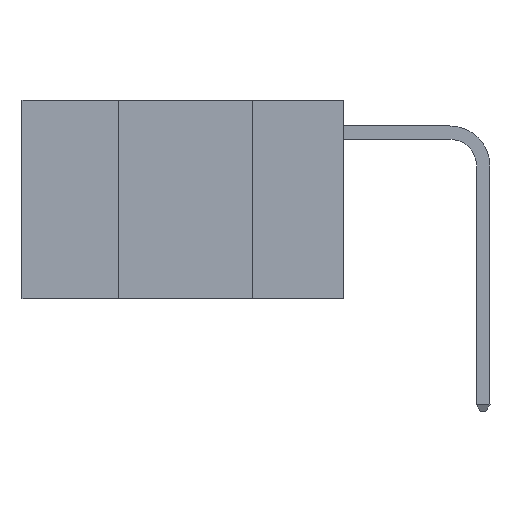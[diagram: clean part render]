
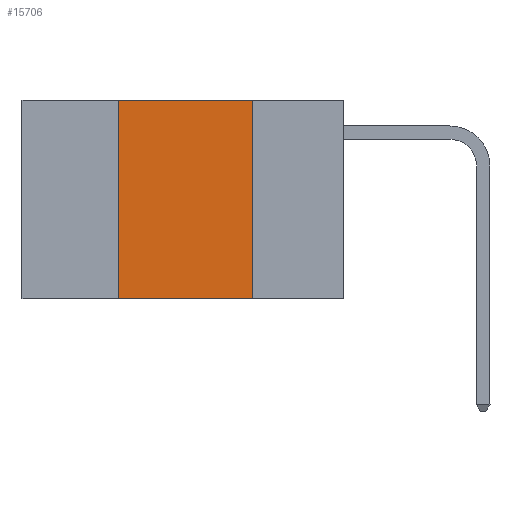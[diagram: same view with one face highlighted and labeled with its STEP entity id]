
A CAD part, left-side view. The second image highlights one B-rep face of the part: STEP entity #15706.
In plain terms, the highlighted planar face has unit normal (-1, 0, 0).
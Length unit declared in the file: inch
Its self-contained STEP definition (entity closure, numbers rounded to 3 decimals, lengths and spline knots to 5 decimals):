
#276 = DIRECTION ( 'NONE',  ( 0., 0., -1. ) ) ;
#886 = CARTESIAN_POINT ( 'NONE',  ( 0., 0.42, 0. ) ) ;
#909 = EDGE_LOOP ( 'NONE', ( #3582, #3209, #13281, #2622 ) ) ;
#1167 = DIRECTION ( 'NONE',  ( 0., -1., 0. ) ) ;
#1270 = LINE ( 'NONE', #5853, #17701 ) ;
#1848 = EDGE_CURVE ( 'NONE', #11623, #16429, #11668, .T. ) ;
#2243 = DIRECTION ( 'NONE',  ( 1., 0., 0. ) ) ;
#2622 = ORIENTED_EDGE ( 'NONE', *, *, #12399, .T. ) ;
#3209 = ORIENTED_EDGE ( 'NONE', *, *, #17516, .F. ) ;
#3312 = VECTOR ( 'NONE', #17788, 39.37008 ) ;
#3582 = ORIENTED_EDGE ( 'NONE', *, *, #1848, .F. ) ;
#3611 = VERTEX_POINT ( 'NONE', #13261 ) ;
#3947 = DIRECTION ( 'NONE',  ( 0., -1., 0. ) ) ;
#4261 = VERTEX_POINT ( 'NONE', #16293 ) ;
#5853 = CARTESIAN_POINT ( 'NONE',  ( 0., 0.6, -0.37 ) ) ;
#7115 = LINE ( 'NONE', #8415, #8289 ) ;
#8156 = DIRECTION ( 'NONE',  ( 0., 0., 1. ) ) ;
#8289 = VECTOR ( 'NONE', #3947, 39.37008 ) ;
#8415 = CARTESIAN_POINT ( 'NONE',  ( 0., 0.6, 0. ) ) ;
#10558 = CARTESIAN_POINT ( 'NONE',  ( 0., 0.17, -0.37 ) ) ;
#11623 = VERTEX_POINT ( 'NONE', #15653 ) ;
#11668 = LINE ( 'NONE', #19071, #3312 ) ;
#11717 = AXIS2_PLACEMENT_3D ( 'NONE', #13834, #2243, #276 ) ;
#12399 = EDGE_CURVE ( 'NONE', #3611, #16429, #1270, .T. ) ;
#13261 = CARTESIAN_POINT ( 'NONE',  ( 0., 0.42, -0.37 ) ) ;
#13281 = ORIENTED_EDGE ( 'NONE', *, *, #19465, .F. ) ;
#13834 = CARTESIAN_POINT ( 'NONE',  ( 0., 0.6, 0. ) ) ;
#15653 = CARTESIAN_POINT ( 'NONE',  ( 0., 0.17, 0. ) ) ;
#15706 = ADVANCED_FACE ( 'NONE', ( #15889 ), #16940, .F. ) ;
#15889 = FACE_OUTER_BOUND ( 'NONE', #909, .T. ) ;
#16293 = CARTESIAN_POINT ( 'NONE',  ( 0., 0.42, 0. ) ) ;
#16429 = VERTEX_POINT ( 'NONE', #10558 ) ;
#16940 = PLANE ( 'NONE',  #11717 ) ;
#17516 = EDGE_CURVE ( 'NONE', #4261, #11623, #7115, .T. ) ;
#17701 = VECTOR ( 'NONE', #1167, 39.37008 ) ;
#17742 = LINE ( 'NONE', #886, #19440 ) ;
#17788 = DIRECTION ( 'NONE',  ( 0., 0., -1. ) ) ;
#19071 = CARTESIAN_POINT ( 'NONE',  ( 0., 0.17, 0. ) ) ;
#19440 = VECTOR ( 'NONE', #8156, 39.37008 ) ;
#19465 = EDGE_CURVE ( 'NONE', #3611, #4261, #17742, .T. ) ;
